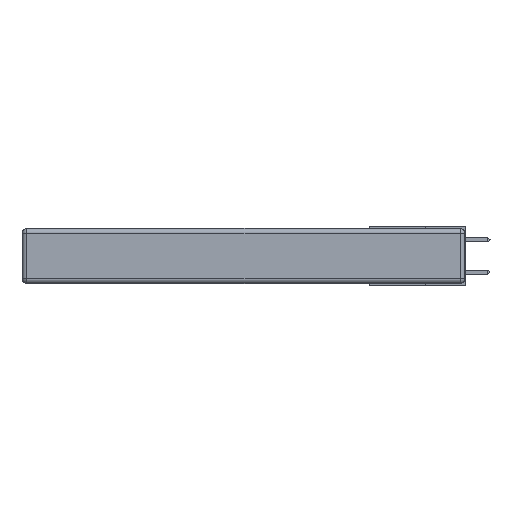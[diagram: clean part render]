
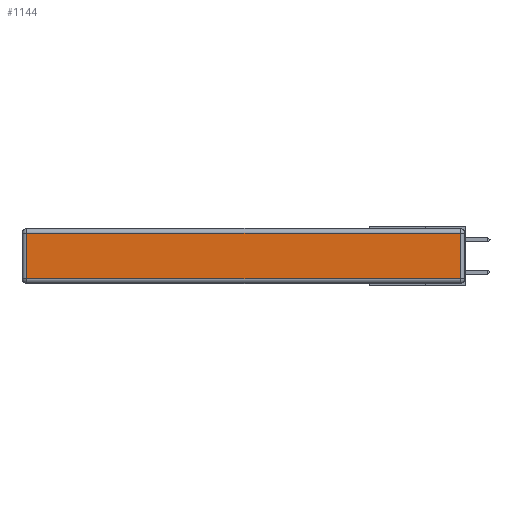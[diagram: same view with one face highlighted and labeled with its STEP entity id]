
A CAD part, left-side view. The second image highlights one B-rep face of the part: STEP entity #1144.
In plain terms, the highlighted planar face has unit normal (-1, 0, 0).
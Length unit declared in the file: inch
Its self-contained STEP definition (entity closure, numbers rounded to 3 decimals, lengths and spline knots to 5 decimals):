
#212 = ORIENTED_EDGE ( 'NONE', *, *, #17418, .T. ) ;
#1144 = ADVANCED_FACE ( 'NONE', ( #13875 ), #29069, .T. ) ;
#1870 = VECTOR ( 'NONE', #26134, 39.37008 ) ;
#4652 = EDGE_LOOP ( 'NONE', ( #24411, #18642, #8533, #212 ) ) ;
#4755 = VECTOR ( 'NONE', #12626, 39.37008 ) ;
#5803 = EDGE_CURVE ( 'NONE', #19239, #7355, #15112, .T. ) ;
#5816 = AXIS2_PLACEMENT_3D ( 'NONE', #6870, #11838, #29190 ) ;
#6870 = CARTESIAN_POINT ( 'NONE',  ( 0., 0., -0.343 ) ) ;
#7291 = EDGE_CURVE ( 'NONE', #24078, #19239, #7666, .T. ) ;
#7355 = VERTEX_POINT ( 'NONE', #14230 ) ;
#7666 = LINE ( 'NONE', #27295, #15388 ) ;
#7737 = CARTESIAN_POINT ( 'NONE',  ( 0., 2.75, -0.03 ) ) ;
#8533 = ORIENTED_EDGE ( 'NONE', *, *, #26637, .T. ) ;
#10913 = CARTESIAN_POINT ( 'NONE',  ( 0., 2.72, -0.313 ) ) ;
#11338 = LINE ( 'NONE', #7737, #4755 ) ;
#11838 = DIRECTION ( 'NONE',  ( -1., 0., 0. ) ) ;
#12439 = DIRECTION ( 'NONE',  ( 0., -1., 0. ) ) ;
#12626 = DIRECTION ( 'NONE',  ( 0., 1., 0. ) ) ;
#13541 = VECTOR ( 'NONE', #27608, 39.37008 ) ;
#13875 = FACE_OUTER_BOUND ( 'NONE', #4652, .T. ) ;
#14230 = CARTESIAN_POINT ( 'NONE',  ( 0., 0.03, -0.03 ) ) ;
#15112 = LINE ( 'NONE', #17898, #13541 ) ;
#15388 = VECTOR ( 'NONE', #12439, 39.37008 ) ;
#17418 = EDGE_CURVE ( 'NONE', #29207, #24078, #30220, .T. ) ;
#17898 = CARTESIAN_POINT ( 'NONE',  ( 0., 0.03, -0.343 ) ) ;
#18642 = ORIENTED_EDGE ( 'NONE', *, *, #5803, .T. ) ;
#19239 = VERTEX_POINT ( 'NONE', #22406 ) ;
#22406 = CARTESIAN_POINT ( 'NONE',  ( 0., 0.03, -0.313 ) ) ;
#23031 = CARTESIAN_POINT ( 'NONE',  ( 0., 2.72, -0.03 ) ) ;
#24078 = VERTEX_POINT ( 'NONE', #10913 ) ;
#24411 = ORIENTED_EDGE ( 'NONE', *, *, #7291, .T. ) ;
#26134 = DIRECTION ( 'NONE',  ( 0., 0., -1. ) ) ;
#26637 = EDGE_CURVE ( 'NONE', #7355, #29207, #11338, .T. ) ;
#27295 = CARTESIAN_POINT ( 'NONE',  ( 0., 0., -0.313 ) ) ;
#27608 = DIRECTION ( 'NONE',  ( 0., 0., 1. ) ) ;
#29069 = PLANE ( 'NONE',  #5816 ) ;
#29190 = DIRECTION ( 'NONE',  ( 0., 0., 1. ) ) ;
#29207 = VERTEX_POINT ( 'NONE', #23031 ) ;
#30220 = LINE ( 'NONE', #31644, #1870 ) ;
#31644 = CARTESIAN_POINT ( 'NONE',  ( 0., 2.72, -0.343 ) ) ;
